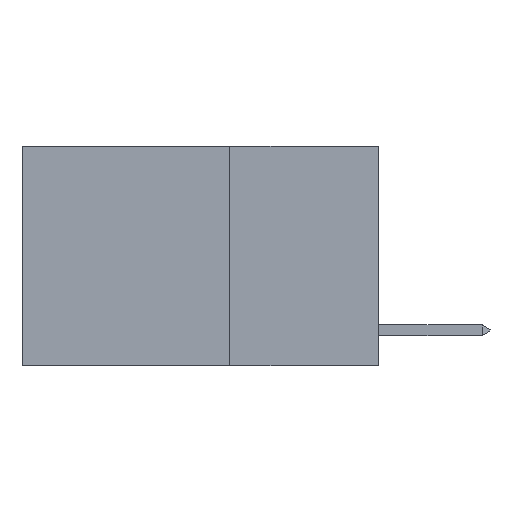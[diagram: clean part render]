
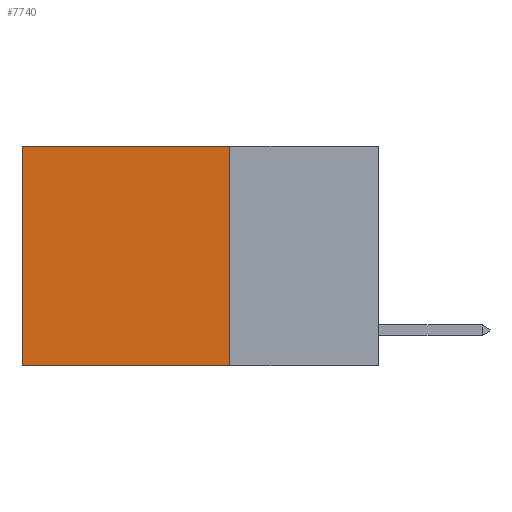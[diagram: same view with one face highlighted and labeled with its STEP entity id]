
A CAD part, left-side view. The second image highlights one B-rep face of the part: STEP entity #7740.
In plain terms, the highlighted planar face has unit normal (-1, 0, 0).
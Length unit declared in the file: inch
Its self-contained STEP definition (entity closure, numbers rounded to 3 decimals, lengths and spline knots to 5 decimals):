
#475 = EDGE_CURVE ( 'NONE', #8235, #7950, #1962, .T. ) ;
#643 = LINE ( 'NONE', #7109, #8081 ) ;
#1088 = ORIENTED_EDGE ( 'NONE', *, *, #475, .F. ) ;
#1427 = CARTESIAN_POINT ( 'NONE',  ( 0.2625, 0.25, 0. ) ) ;
#1676 = DIRECTION ( 'NONE',  ( 1., 0., 0. ) ) ;
#1962 = LINE ( 'NONE', #1427, #10361 ) ;
#2434 = CARTESIAN_POINT ( 'NONE',  ( 0.2625, 0.25, 0. ) ) ;
#2764 = EDGE_CURVE ( 'NONE', #7950, #2941, #643, .T. ) ;
#2782 = DIRECTION ( 'NONE',  ( 0., 1., 0. ) ) ;
#2785 = EDGE_CURVE ( 'NONE', #8235, #13399, #8475, .T. ) ;
#2941 = VERTEX_POINT ( 'NONE', #15830 ) ;
#3347 = VECTOR ( 'NONE', #12310, 39.37008 ) ;
#4085 = PLANE ( 'NONE',  #12032 ) ;
#4362 = CARTESIAN_POINT ( 'NONE',  ( 0.2625, 0.25, -0.37 ) ) ;
#5249 = DIRECTION ( 'NONE',  ( 0., 0., -1. ) ) ;
#5289 = CARTESIAN_POINT ( 'NONE',  ( 0.2625, 0.25, 0. ) ) ;
#6898 = ORIENTED_EDGE ( 'NONE', *, *, #2785, .T. ) ;
#7109 = CARTESIAN_POINT ( 'NONE',  ( 0.2625, 0.25, -0.37 ) ) ;
#7531 = CARTESIAN_POINT ( 'NONE',  ( 0.2625, 0.6, 0. ) ) ;
#7740 = ADVANCED_FACE ( 'NONE', ( #14298 ), #4085, .F. ) ;
#7835 = DIRECTION ( 'NONE',  ( 0., 0., -1. ) ) ;
#7950 = VERTEX_POINT ( 'NONE', #4362 ) ;
#8081 = VECTOR ( 'NONE', #12425, 39.37008 ) ;
#8235 = VERTEX_POINT ( 'NONE', #2434 ) ;
#8475 = LINE ( 'NONE', #5289, #13758 ) ;
#10166 = ORIENTED_EDGE ( 'NONE', *, *, #2764, .F. ) ;
#10361 = VECTOR ( 'NONE', #5249, 39.37008 ) ;
#12032 = AXIS2_PLACEMENT_3D ( 'NONE', #12998, #1676, #7835 ) ;
#12310 = DIRECTION ( 'NONE',  ( 0., 0., -1. ) ) ;
#12425 = DIRECTION ( 'NONE',  ( 0., 1., 0. ) ) ;
#12499 = EDGE_LOOP ( 'NONE', ( #13144, #10166, #1088, #6898 ) ) ;
#12619 = CARTESIAN_POINT ( 'NONE',  ( 0.2625, 0.6, 0. ) ) ;
#12998 = CARTESIAN_POINT ( 'NONE',  ( 0.2625, 0.25, 0. ) ) ;
#13144 = ORIENTED_EDGE ( 'NONE', *, *, #13745, .T. ) ;
#13399 = VERTEX_POINT ( 'NONE', #12619 ) ;
#13745 = EDGE_CURVE ( 'NONE', #13399, #2941, #15667, .T. ) ;
#13758 = VECTOR ( 'NONE', #2782, 39.37008 ) ;
#14298 = FACE_OUTER_BOUND ( 'NONE', #12499, .T. ) ;
#15667 = LINE ( 'NONE', #7531, #3347 ) ;
#15830 = CARTESIAN_POINT ( 'NONE',  ( 0.2625, 0.6, -0.37 ) ) ;
